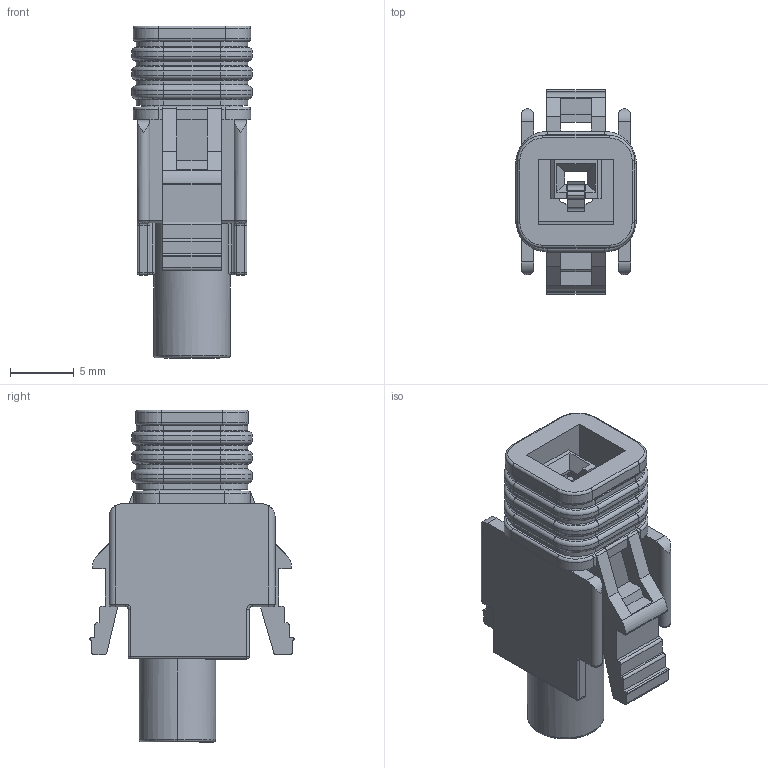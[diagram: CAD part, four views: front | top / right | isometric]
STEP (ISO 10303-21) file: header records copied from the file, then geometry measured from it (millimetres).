
FILE_DESCRIPTION (( 'STEP AP214' ), '1' );
FILE_NAME ('572-001-000-400.STEP', '2020-07-30T16:25:03', ( '' ), ( '' ), 'SwSTEP 2.0', 'SolidWorks 2020', '' );
FILE_SCHEMA (( 'AUTOMOTIVE_DESIGN' ));
Length unit declared in the file: millimetre
Products named in the file (3): 572-001-000-FEMALE-HOUSING_BLUE; 570-001-000-HOUSING-SEAL; 572-001-000-400
Assembly tree (2 placements, depth 2):
  572-001-000-400
    572-001-000-FEMALE-HOUSING_BLUE
    570-001-000-HOUSING-SEAL
Bounding box: 9.45 x 16 x 26 mm (x, y, z)
Volume: 1238.1 mm3; surface area: 2576.9 mm2
Topology: 2 solids, 2 shells, 633 faces, 1512 edges, 875 vertices
Faces by surface type: cylinder 264, plane 228, torus 125, sphere 8, bspline 5, cone 3
Entity records: 18320 total; most frequent: CARTESIAN_POINT 3352, DIRECTION 3339, ORIENTED_EDGE 3008, EDGE_CURVE 1504, AXIS2_PLACEMENT_3D 1245, VERTEX_POINT 875, VECTOR 849, LINE 849
